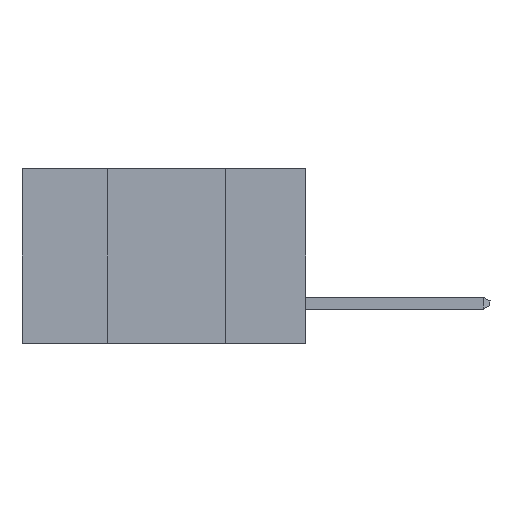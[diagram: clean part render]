
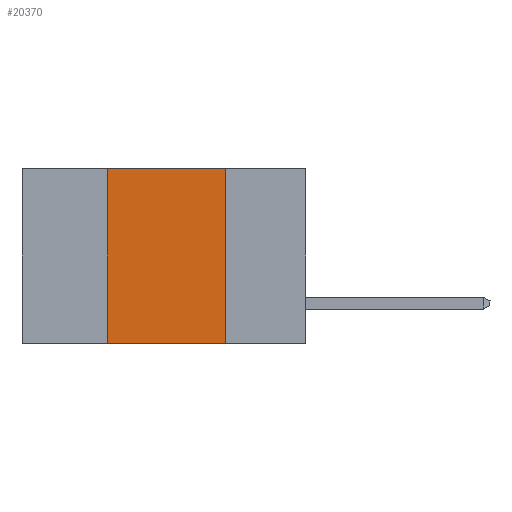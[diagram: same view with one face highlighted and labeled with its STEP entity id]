
A CAD part, left-side view. The second image highlights one B-rep face of the part: STEP entity #20370.
In plain terms, the highlighted planar face has unit normal (-1, 0, 0).
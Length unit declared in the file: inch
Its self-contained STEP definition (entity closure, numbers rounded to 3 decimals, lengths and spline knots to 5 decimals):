
#934 = LINE ( 'NONE', #17695, #5626 ) ;
#1827 = VERTEX_POINT ( 'NONE', #16003 ) ;
#2828 = CARTESIAN_POINT ( 'NONE',  ( 0., 0.42, -0.37 ) ) ;
#3370 = AXIS2_PLACEMENT_3D ( 'NONE', #9220, #12808, #14701 ) ;
#5032 = ORIENTED_EDGE ( 'NONE', *, *, #18642, .T. ) ;
#5626 = VECTOR ( 'NONE', #23202, 39.37008 ) ;
#5732 = PLANE ( 'NONE',  #3370 ) ;
#6233 = ORIENTED_EDGE ( 'NONE', *, *, #7691, .F. ) ;
#7026 = VECTOR ( 'NONE', #23632, 39.37008 ) ;
#7691 = EDGE_CURVE ( 'NONE', #8800, #1827, #16347, .T. ) ;
#8185 = CARTESIAN_POINT ( 'NONE',  ( 0., 0.17, -0.37 ) ) ;
#8627 = VECTOR ( 'NONE', #11778, 39.37008 ) ;
#8800 = VERTEX_POINT ( 'NONE', #21385 ) ;
#9220 = CARTESIAN_POINT ( 'NONE',  ( 0., 0.6, 0. ) ) ;
#10094 = EDGE_CURVE ( 'NONE', #14641, #8800, #13967, .T. ) ;
#10196 = CARTESIAN_POINT ( 'NONE',  ( 0., 0.42, -0.37 ) ) ;
#11410 = VERTEX_POINT ( 'NONE', #19164 ) ;
#11593 = ORIENTED_EDGE ( 'NONE', *, *, #10094, .F. ) ;
#11778 = DIRECTION ( 'NONE',  ( 0., 0., -1. ) ) ;
#12113 = EDGE_LOOP ( 'NONE', ( #18762, #6233, #11593, #5032 ) ) ;
#12660 = CARTESIAN_POINT ( 'NONE',  ( 0., 0.6, 0. ) ) ;
#12808 = DIRECTION ( 'NONE',  ( 1., 0., 0. ) ) ;
#13967 = LINE ( 'NONE', #2828, #22666 ) ;
#14337 = EDGE_CURVE ( 'NONE', #1827, #11410, #22998, .T. ) ;
#14641 = VERTEX_POINT ( 'NONE', #10196 ) ;
#14701 = DIRECTION ( 'NONE',  ( 0., 0., -1. ) ) ;
#16003 = CARTESIAN_POINT ( 'NONE',  ( 0., 0.17, 0. ) ) ;
#16347 = LINE ( 'NONE', #12660, #7026 ) ;
#17695 = CARTESIAN_POINT ( 'NONE',  ( 0., 0.6, -0.37 ) ) ;
#18642 = EDGE_CURVE ( 'NONE', #14641, #11410, #934, .T. ) ;
#18762 = ORIENTED_EDGE ( 'NONE', *, *, #14337, .F. ) ;
#19164 = CARTESIAN_POINT ( 'NONE',  ( 0., 0.17, -0.37 ) ) ;
#20370 = ADVANCED_FACE ( 'NONE', ( #21880 ), #5732, .F. ) ;
#21154 = DIRECTION ( 'NONE',  ( 0., 0., 1. ) ) ;
#21385 = CARTESIAN_POINT ( 'NONE',  ( 0., 0.42, 0. ) ) ;
#21880 = FACE_OUTER_BOUND ( 'NONE', #12113, .T. ) ;
#22666 = VECTOR ( 'NONE', #21154, 39.37008 ) ;
#22998 = LINE ( 'NONE', #8185, #8627 ) ;
#23202 = DIRECTION ( 'NONE',  ( 0., -1., 0. ) ) ;
#23632 = DIRECTION ( 'NONE',  ( 0., -1., 0. ) ) ;
